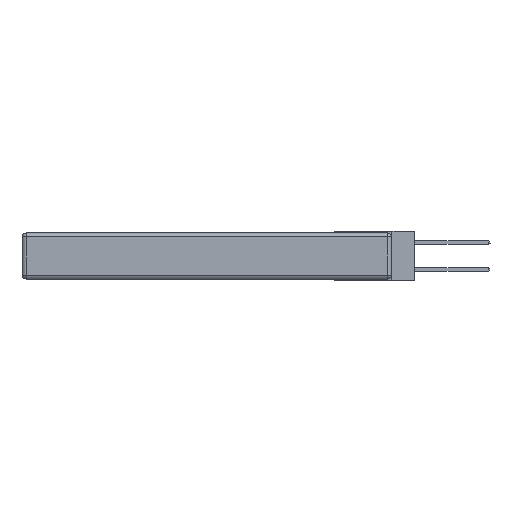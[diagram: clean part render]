
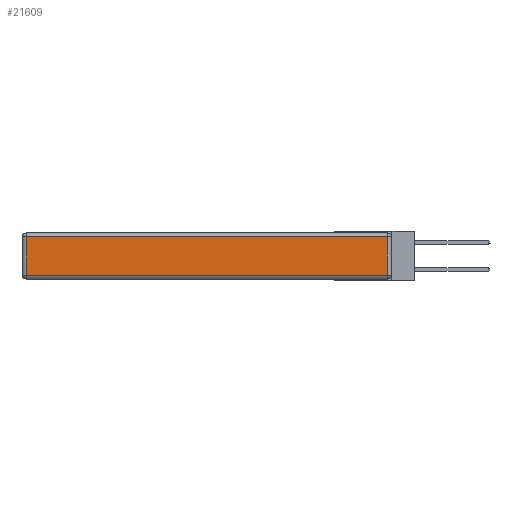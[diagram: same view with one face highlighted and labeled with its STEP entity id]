
A CAD part, left-side view. The second image highlights one B-rep face of the part: STEP entity #21609.
In plain terms, the highlighted planar face has unit normal (-1, 0, 0).
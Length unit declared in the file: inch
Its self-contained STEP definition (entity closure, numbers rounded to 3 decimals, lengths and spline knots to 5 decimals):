
#181 = LINE ( 'NONE', #12119, #18718 ) ;
#847 = CARTESIAN_POINT ( 'NONE',  ( 0., 2.72, -0.313 ) ) ;
#2396 = DIRECTION ( 'NONE',  ( -1., 0., 0. ) ) ;
#4153 = CARTESIAN_POINT ( 'NONE',  ( 0., 0.03, -0.03 ) ) ;
#4442 = VECTOR ( 'NONE', #12437, 39.37008 ) ;
#4810 = VERTEX_POINT ( 'NONE', #847 ) ;
#5341 = EDGE_CURVE ( 'NONE', #20586, #4810, #22409, .T. ) ;
#5891 = AXIS2_PLACEMENT_3D ( 'NONE', #9943, #2396, #16742 ) ;
#6818 = DIRECTION ( 'NONE',  ( 0., 1., 0. ) ) ;
#7121 = CARTESIAN_POINT ( 'NONE',  ( 0., 0.03, -0.343 ) ) ;
#7346 = CARTESIAN_POINT ( 'NONE',  ( 0., 2.72, -0.343 ) ) ;
#8135 = PLANE ( 'NONE',  #5891 ) ;
#9095 = VERTEX_POINT ( 'NONE', #22717 ) ;
#9380 = EDGE_LOOP ( 'NONE', ( #19185, #20427, #18239, #12903 ) ) ;
#9943 = CARTESIAN_POINT ( 'NONE',  ( 0., 0., -0.343 ) ) ;
#10592 = EDGE_CURVE ( 'NONE', #4810, #9095, #181, .T. ) ;
#10721 = EDGE_CURVE ( 'NONE', #9095, #22086, #21802, .T. ) ;
#12119 = CARTESIAN_POINT ( 'NONE',  ( 0., 0., -0.313 ) ) ;
#12437 = DIRECTION ( 'NONE',  ( 0., 0., 1. ) ) ;
#12903 = ORIENTED_EDGE ( 'NONE', *, *, #5341, .T. ) ;
#13411 = LINE ( 'NONE', #20948, #17072 ) ;
#14079 = EDGE_CURVE ( 'NONE', #22086, #20586, #13411, .T. ) ;
#16742 = DIRECTION ( 'NONE',  ( 0., 0., 1. ) ) ;
#17072 = VECTOR ( 'NONE', #6818, 39.37008 ) ;
#17729 = CARTESIAN_POINT ( 'NONE',  ( 0., 2.72, -0.03 ) ) ;
#18239 = ORIENTED_EDGE ( 'NONE', *, *, #14079, .T. ) ;
#18718 = VECTOR ( 'NONE', #21170, 39.37008 ) ;
#19185 = ORIENTED_EDGE ( 'NONE', *, *, #10592, .T. ) ;
#20427 = ORIENTED_EDGE ( 'NONE', *, *, #10721, .T. ) ;
#20586 = VERTEX_POINT ( 'NONE', #17729 ) ;
#20948 = CARTESIAN_POINT ( 'NONE',  ( 0., 2.75, -0.03 ) ) ;
#21170 = DIRECTION ( 'NONE',  ( 0., -1., 0. ) ) ;
#21555 = DIRECTION ( 'NONE',  ( 0., 0., -1. ) ) ;
#21581 = VECTOR ( 'NONE', #21555, 39.37008 ) ;
#21609 = ADVANCED_FACE ( 'NONE', ( #22187 ), #8135, .T. ) ;
#21802 = LINE ( 'NONE', #7121, #4442 ) ;
#22086 = VERTEX_POINT ( 'NONE', #4153 ) ;
#22187 = FACE_OUTER_BOUND ( 'NONE', #9380, .T. ) ;
#22409 = LINE ( 'NONE', #7346, #21581 ) ;
#22717 = CARTESIAN_POINT ( 'NONE',  ( 0., 0.03, -0.313 ) ) ;
